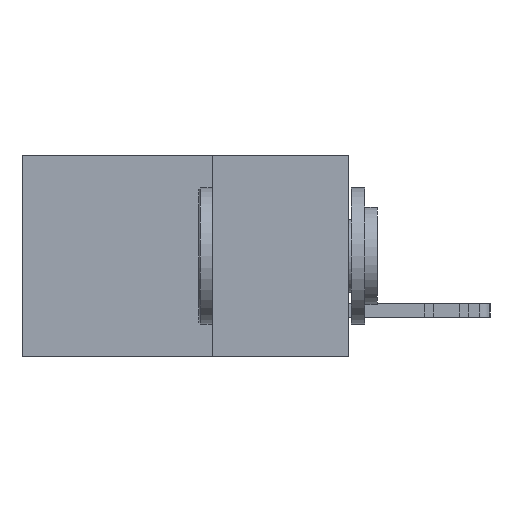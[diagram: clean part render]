
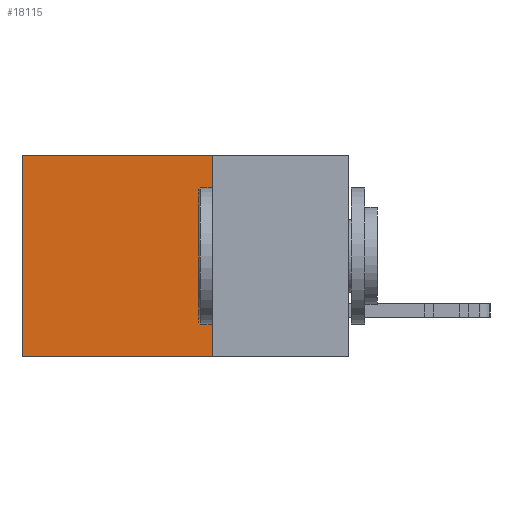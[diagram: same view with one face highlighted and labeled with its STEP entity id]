
A CAD part, left-side view. The second image highlights one B-rep face of the part: STEP entity #18115.
In plain terms, the highlighted planar face has unit normal (-1, 0, 0).
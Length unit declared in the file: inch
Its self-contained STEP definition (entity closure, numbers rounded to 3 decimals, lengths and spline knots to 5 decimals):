
#456 = CARTESIAN_POINT ( 'NONE',  ( 0.2615, 0.25, -0.37 ) ) ;
#916 = EDGE_LOOP ( 'NONE', ( #4083, #13161, #4787, #1575 ) ) ;
#1447 = DIRECTION ( 'NONE',  ( 0., 0., -1. ) ) ;
#1575 = ORIENTED_EDGE ( 'NONE', *, *, #14866, .T. ) ;
#2014 = LINE ( 'NONE', #17952, #2636 ) ;
#2634 = LINE ( 'NONE', #23181, #12309 ) ;
#2636 = VECTOR ( 'NONE', #4574, 39.37008 ) ;
#2979 = EDGE_CURVE ( 'NONE', #5046, #9004, #8688, .T. ) ;
#3558 = FACE_OUTER_BOUND ( 'NONE', #916, .T. ) ;
#3659 = CARTESIAN_POINT ( 'NONE',  ( 0.2615, 0.6, -0.37 ) ) ;
#3930 = EDGE_CURVE ( 'NONE', #20819, #5046, #2634, .T. ) ;
#4083 = ORIENTED_EDGE ( 'NONE', *, *, #17930, .T. ) ;
#4574 = DIRECTION ( 'NONE',  ( 0., 0., -1. ) ) ;
#4787 = ORIENTED_EDGE ( 'NONE', *, *, #3930, .F. ) ;
#5023 = VECTOR ( 'NONE', #16790, 39.37008 ) ;
#5046 = VERTEX_POINT ( 'NONE', #456 ) ;
#5878 = CARTESIAN_POINT ( 'NONE',  ( 0.2615, 0.6, 0. ) ) ;
#8688 = LINE ( 'NONE', #9572, #18899 ) ;
#8935 = DIRECTION ( 'NONE',  ( 0., 1., 0. ) ) ;
#9004 = VERTEX_POINT ( 'NONE', #3659 ) ;
#9572 = CARTESIAN_POINT ( 'NONE',  ( 0.2615, 0.25, -0.37 ) ) ;
#10105 = LINE ( 'NONE', #24281, #5023 ) ;
#10456 = VERTEX_POINT ( 'NONE', #5878 ) ;
#12309 = VECTOR ( 'NONE', #23146, 39.37008 ) ;
#13031 = DIRECTION ( 'NONE',  ( 1., 0., 0. ) ) ;
#13161 = ORIENTED_EDGE ( 'NONE', *, *, #2979, .F. ) ;
#14866 = EDGE_CURVE ( 'NONE', #20819, #10456, #10105, .T. ) ;
#16773 = PLANE ( 'NONE',  #18319 ) ;
#16790 = DIRECTION ( 'NONE',  ( 0., 1., 0. ) ) ;
#17930 = EDGE_CURVE ( 'NONE', #10456, #9004, #2014, .T. ) ;
#17952 = CARTESIAN_POINT ( 'NONE',  ( 0.2615, 0.6, -0.37 ) ) ;
#18115 = ADVANCED_FACE ( 'NONE', ( #3558 ), #16773, .F. ) ;
#18319 = AXIS2_PLACEMENT_3D ( 'NONE', #24349, #13031, #1447 ) ;
#18666 = CARTESIAN_POINT ( 'NONE',  ( 0.2615, 0.25, 0. ) ) ;
#18899 = VECTOR ( 'NONE', #8935, 39.37008 ) ;
#20819 = VERTEX_POINT ( 'NONE', #18666 ) ;
#23146 = DIRECTION ( 'NONE',  ( 0., 0., -1. ) ) ;
#23181 = CARTESIAN_POINT ( 'NONE',  ( 0.2615, 0.25, -0.37 ) ) ;
#24281 = CARTESIAN_POINT ( 'NONE',  ( 0.2615, 0.25, 0. ) ) ;
#24349 = CARTESIAN_POINT ( 'NONE',  ( 0.2615, 0.25, -0.37 ) ) ;
